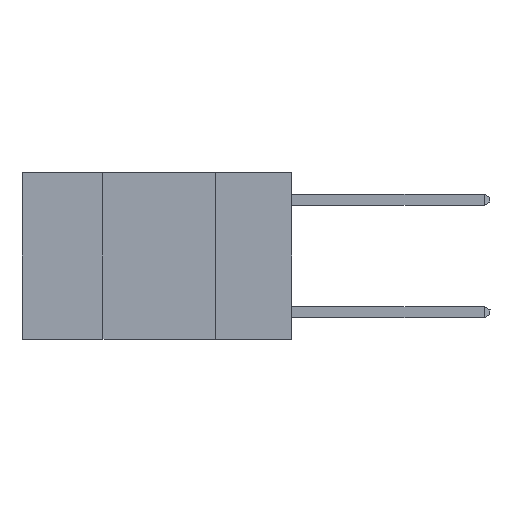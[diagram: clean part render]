
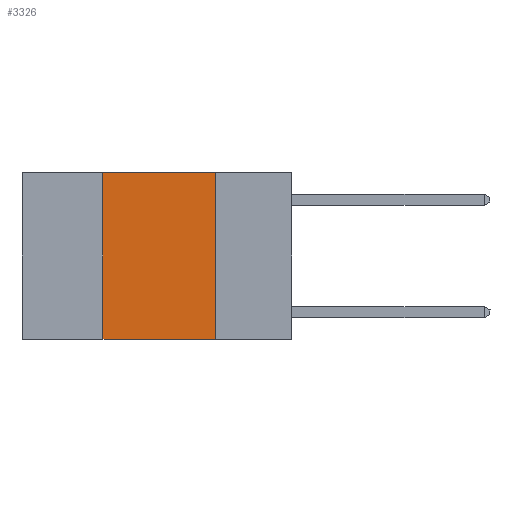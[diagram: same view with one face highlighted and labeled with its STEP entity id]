
A CAD part, left-side view. The second image highlights one B-rep face of the part: STEP entity #3326.
In plain terms, the highlighted planar face has unit normal (-1, 0, 0).
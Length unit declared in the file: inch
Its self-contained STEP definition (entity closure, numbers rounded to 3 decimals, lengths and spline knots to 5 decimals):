
#431 = VERTEX_POINT ( 'NONE', #6337 ) ;
#574 = EDGE_CURVE ( 'NONE', #10029, #10640, #8153, .T. ) ;
#689 = CARTESIAN_POINT ( 'NONE',  ( 0., 0.42, -0.37 ) ) ;
#699 = FACE_OUTER_BOUND ( 'NONE', #2162, .T. ) ;
#1099 = VECTOR ( 'NONE', #11379, 39.37008 ) ;
#1503 = CARTESIAN_POINT ( 'NONE',  ( 0., 0.42, 0. ) ) ;
#1983 = VECTOR ( 'NONE', #8099, 39.37008 ) ;
#2162 = EDGE_LOOP ( 'NONE', ( #5559, #11415, #9308, #5524 ) ) ;
#2271 = VECTOR ( 'NONE', #4978, 39.37008 ) ;
#2927 = EDGE_CURVE ( 'NONE', #10029, #10750, #6986, .T. ) ;
#2998 = LINE ( 'NONE', #3159, #7132 ) ;
#3088 = DIRECTION ( 'NONE',  ( 0., 0., -1. ) ) ;
#3092 = DIRECTION ( 'NONE',  ( 1., 0., 0. ) ) ;
#3152 = PLANE ( 'NONE',  #4495 ) ;
#3159 = CARTESIAN_POINT ( 'NONE',  ( 0., 0.6, 0. ) ) ;
#3326 = ADVANCED_FACE ( 'NONE', ( #699 ), #3152, .F. ) ;
#3959 = CARTESIAN_POINT ( 'NONE',  ( 0., 0.6, 0. ) ) ;
#4495 = AXIS2_PLACEMENT_3D ( 'NONE', #3959, #3092, #3088 ) ;
#4978 = DIRECTION ( 'NONE',  ( 0., 0., -1. ) ) ;
#5524 = ORIENTED_EDGE ( 'NONE', *, *, #2927, .T. ) ;
#5559 = ORIENTED_EDGE ( 'NONE', *, *, #10514, .F. ) ;
#6337 = CARTESIAN_POINT ( 'NONE',  ( 0., 0.17, 0. ) ) ;
#6686 = CARTESIAN_POINT ( 'NONE',  ( 0., 0.17, 0. ) ) ;
#6732 = DIRECTION ( 'NONE',  ( 0., -1., 0. ) ) ;
#6986 = LINE ( 'NONE', #7837, #1983 ) ;
#6998 = CARTESIAN_POINT ( 'NONE',  ( 0., 0.17, -0.37 ) ) ;
#7132 = VECTOR ( 'NONE', #6732, 39.37008 ) ;
#7252 = LINE ( 'NONE', #6686, #2271 ) ;
#7837 = CARTESIAN_POINT ( 'NONE',  ( 0., 0.6, -0.37 ) ) ;
#8099 = DIRECTION ( 'NONE',  ( 0., -1., 0. ) ) ;
#8153 = LINE ( 'NONE', #11331, #1099 ) ;
#9308 = ORIENTED_EDGE ( 'NONE', *, *, #574, .F. ) ;
#9845 = EDGE_CURVE ( 'NONE', #10640, #431, #2998, .T. ) ;
#10029 = VERTEX_POINT ( 'NONE', #689 ) ;
#10514 = EDGE_CURVE ( 'NONE', #431, #10750, #7252, .T. ) ;
#10640 = VERTEX_POINT ( 'NONE', #1503 ) ;
#10750 = VERTEX_POINT ( 'NONE', #6998 ) ;
#11331 = CARTESIAN_POINT ( 'NONE',  ( 0., 0.42, 0. ) ) ;
#11379 = DIRECTION ( 'NONE',  ( 0., 0., 1. ) ) ;
#11415 = ORIENTED_EDGE ( 'NONE', *, *, #9845, .F. ) ;
